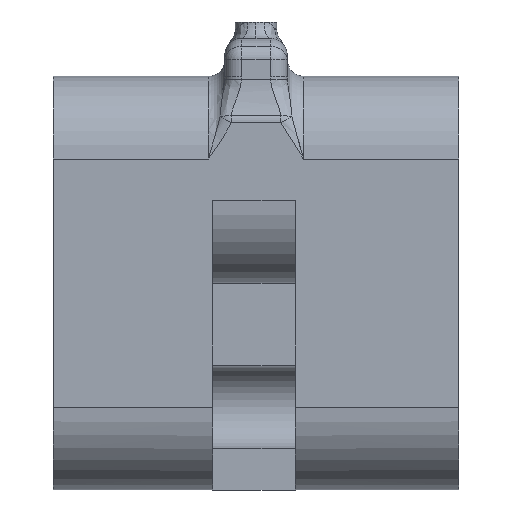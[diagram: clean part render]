
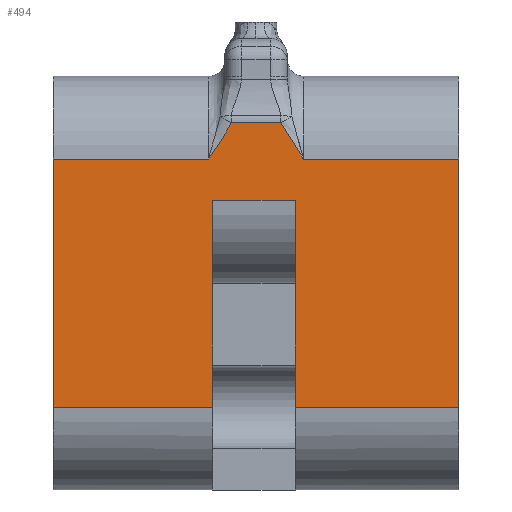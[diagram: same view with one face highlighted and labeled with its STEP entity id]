
A CAD part, front view. The second image highlights one B-rep face of the part: STEP entity #494.
In plain terms, the highlighted planar face has unit normal (0, -1, 0).
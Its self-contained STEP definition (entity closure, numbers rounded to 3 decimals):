
#110 = CARTESIAN_POINT ( 'NONE',  ( 28.243, -10., 32.181 ) ) ;
#115 = VERTEX_POINT ( 'NONE', #1654 ) ;
#188 = CARTESIAN_POINT ( 'NONE',  ( 49., -10., 29.345 ) ) ;
#259 = EDGE_CURVE ( 'NONE', #1880, #4710, #4178, .T. ) ;
#390 = CARTESIAN_POINT ( 'NONE',  ( 19.25, -10., -0.655 ) ) ;
#406 = DIRECTION ( 'NONE',  ( 0., 0., -1. ) ) ;
#482 = CARTESIAN_POINT ( 'NONE',  ( 30.25, -10., 29.345 ) ) ;
#494 = ADVANCED_FACE ( 'NONE', ( #1255 ), #2719, .F. ) ;
#531 = DIRECTION ( 'NONE',  ( -1., 0., 0. ) ) ;
#641 = CARTESIAN_POINT ( 'NONE',  ( 18.75, -10., 29.345 ) ) ;
#656 = CARTESIAN_POINT ( 'NONE',  ( 19.25, -10., 14.345 ) ) ;
#669 = VERTEX_POINT ( 'NONE', #2231 ) ;
#671 = ORIENTED_EDGE ( 'NONE', *, *, #1751, .T. ) ;
#687 = ORIENTED_EDGE ( 'NONE', *, *, #1184, .F. ) ;
#701 = ORIENTED_EDGE ( 'NONE', *, *, #1715, .F. ) ;
#867 = CARTESIAN_POINT ( 'NONE',  ( 29.25, -10., 14.345 ) ) ;
#896 = VECTOR ( 'NONE', #406, 1000. ) ;
#1102 = LINE ( 'NONE', #3932, #2811 ) ;
#1156 = LINE ( 'NONE', #2899, #1277 ) ;
#1184 = EDGE_CURVE ( 'NONE', #669, #2606, #2725, .T. ) ;
#1230 = CARTESIAN_POINT ( 'NONE',  ( 30.25, -10., 29.345 ) ) ;
#1255 = FACE_OUTER_BOUND ( 'NONE', #4703, .T. ) ;
#1276 = CARTESIAN_POINT ( 'NONE',  ( 49., -10., -0.655 ) ) ;
#1277 = VECTOR ( 'NONE', #3592, 1000. ) ;
#1285 = ORIENTED_EDGE ( 'NONE', *, *, #1675, .T. ) ;
#1381 = CARTESIAN_POINT ( 'NONE',  ( 21.527, -10., 33.727 ) ) ;
#1405 = CARTESIAN_POINT ( 'NONE',  ( 49., -10., 29.345 ) ) ;
#1433 = EDGE_CURVE ( 'NONE', #1954, #3858, #3478, .T. ) ;
#1469 = EDGE_CURVE ( 'NONE', #669, #3858, #2438, .T. ) ;
#1502 = VERTEX_POINT ( 'NONE', #2718 ) ;
#1506 = ORIENTED_EDGE ( 'NONE', *, *, #1469, .T. ) ;
#1568 = VECTOR ( 'NONE', #531, 1000. ) ;
#1599 = EDGE_CURVE ( 'NONE', #1880, #115, #1986, .T. ) ;
#1652 = ORIENTED_EDGE ( 'NONE', *, *, #259, .T. ) ;
#1654 = CARTESIAN_POINT ( 'NONE',  ( 49., -10., -0.655 ) ) ;
#1675 = EDGE_CURVE ( 'NONE', #4710, #4110, #2772, .T. ) ;
#1715 = EDGE_CURVE ( 'NONE', #115, #1954, #4276, .T. ) ;
#1732 = CARTESIAN_POINT ( 'NONE',  ( 21.527, -10., 33.727 ) ) ;
#1736 = VERTEX_POINT ( 'NONE', #3406 ) ;
#1751 = EDGE_CURVE ( 'NONE', #4110, #2814, #2527, .T. ) ;
#1840 = EDGE_CURVE ( 'NONE', #2814, #4041, #2340, .T. ) ;
#1880 = VERTEX_POINT ( 'NONE', #1405 ) ;
#1915 = EDGE_CURVE ( 'NONE', #1736, #1502, #1102, .T. ) ;
#1954 = VERTEX_POINT ( 'NONE', #2559 ) ;
#1981 = DIRECTION ( 'NONE',  ( -1., 0., 0. ) ) ;
#1986 = LINE ( 'NONE', #2986, #896 ) ;
#2076 = LINE ( 'NONE', #4075, #4694 ) ;
#2231 = CARTESIAN_POINT ( 'NONE',  ( 19.25, -10., 24.345 ) ) ;
#2297 = ORIENTED_EDGE ( 'NONE', *, *, #1915, .T. ) ;
#2323 = VECTOR ( 'NONE', #3401, 1000. ) ;
#2340 = B_SPLINE_CURVE_WITH_KNOTS ( 'NONE', 3,
 ( #1732, #3876, #2825, #641 ),
 .UNSPECIFIED., .F., .F.,
 ( 4, 4 ),
 ( 0.005, 0.01 ),
 .UNSPECIFIED. ) ;
#2344 = CARTESIAN_POINT ( 'NONE',  ( 49., -10., -0.655 ) ) ;
#2438 = LINE ( 'NONE', #4486, #2323 ) ;
#2483 = ORIENTED_EDGE ( 'NONE', *, *, #1433, .F. ) ;
#2527 = LINE ( 'NONE', #3063, #1568 ) ;
#2546 = VECTOR ( 'NONE', #3385, 1000. ) ;
#2559 = CARTESIAN_POINT ( 'NONE',  ( 29.25, -10., -0.655 ) ) ;
#2567 = CARTESIAN_POINT ( 'NONE',  ( 18.75, -10., 29.345 ) ) ;
#2606 = VERTEX_POINT ( 'NONE', #390 ) ;
#2678 = CARTESIAN_POINT ( 'NONE',  ( 29.248, -10., 30.763 ) ) ;
#2693 = CARTESIAN_POINT ( 'NONE',  ( 27.473, -10., 33.727 ) ) ;
#2718 = CARTESIAN_POINT ( 'NONE',  ( 0., -10., -0.655 ) ) ;
#2719 = PLANE ( 'NONE',  #3271 ) ;
#2725 = LINE ( 'NONE', #656, #4624 ) ;
#2772 = B_SPLINE_CURVE_WITH_KNOTS ( 'NONE', 3,
 ( #1230, #2678, #110, #2693 ),
 .UNSPECIFIED., .F., .F.,
 ( 4, 4 ),
 ( 0., 0.005 ),
 .UNSPECIFIED. ) ;
#2806 = DIRECTION ( 'NONE',  ( 0., 0., 1. ) ) ;
#2811 = VECTOR ( 'NONE', #3561, 1000. ) ;
#2814 = VERTEX_POINT ( 'NONE', #1381 ) ;
#2825 = CARTESIAN_POINT ( 'NONE',  ( 19.753, -10., 30.764 ) ) ;
#2899 = CARTESIAN_POINT ( 'NONE',  ( 49., -10., 29.345 ) ) ;
#2959 = CARTESIAN_POINT ( 'NONE',  ( 27.473, -10., 33.727 ) ) ;
#2986 = CARTESIAN_POINT ( 'NONE',  ( 49., -10., -0.655 ) ) ;
#3063 = CARTESIAN_POINT ( 'NONE',  ( 49., -10., 33.727 ) ) ;
#3106 = VECTOR ( 'NONE', #3388, 1000. ) ;
#3108 = ORIENTED_EDGE ( 'NONE', *, *, #1599, .F. ) ;
#3173 = DIRECTION ( 'NONE',  ( 0., 0., -1. ) ) ;
#3271 = AXIS2_PLACEMENT_3D ( 'NONE', #1276, #4244, #2806 ) ;
#3306 = VECTOR ( 'NONE', #1981, 1000. ) ;
#3385 = DIRECTION ( 'NONE',  ( 0., 0., 1. ) ) ;
#3388 = DIRECTION ( 'NONE',  ( -1., 0., 0. ) ) ;
#3401 = DIRECTION ( 'NONE',  ( 1., 0., 0. ) ) ;
#3406 = CARTESIAN_POINT ( 'NONE',  ( 0., -10., 29.345 ) ) ;
#3430 = CARTESIAN_POINT ( 'NONE',  ( 29.25, -10., 24.345 ) ) ;
#3478 = LINE ( 'NONE', #867, #2546 ) ;
#3505 = ORIENTED_EDGE ( 'NONE', *, *, #4373, .T. ) ;
#3561 = DIRECTION ( 'NONE',  ( 0., 0., -1. ) ) ;
#3592 = DIRECTION ( 'NONE',  ( -1., 0., 0. ) ) ;
#3858 = VERTEX_POINT ( 'NONE', #3430 ) ;
#3876 = CARTESIAN_POINT ( 'NONE',  ( 20.757, -10., 32.181 ) ) ;
#3932 = CARTESIAN_POINT ( 'NONE',  ( 0., -10., -0.655 ) ) ;
#4041 = VERTEX_POINT ( 'NONE', #2567 ) ;
#4075 = CARTESIAN_POINT ( 'NONE',  ( 49., -10., -0.655 ) ) ;
#4110 = VERTEX_POINT ( 'NONE', #2959 ) ;
#4156 = EDGE_CURVE ( 'NONE', #2606, #1502, #2076, .T. ) ;
#4162 = ORIENTED_EDGE ( 'NONE', *, *, #4156, .F. ) ;
#4178 = LINE ( 'NONE', #188, #3106 ) ;
#4244 = DIRECTION ( 'NONE',  ( 0., 1., 0. ) ) ;
#4276 = LINE ( 'NONE', #2344, #3306 ) ;
#4315 = ORIENTED_EDGE ( 'NONE', *, *, #1840, .T. ) ;
#4373 = EDGE_CURVE ( 'NONE', #4041, #1736, #1156, .T. ) ;
#4478 = DIRECTION ( 'NONE',  ( -1., 0., 0. ) ) ;
#4486 = CARTESIAN_POINT ( 'NONE',  ( 49., -10., 24.345 ) ) ;
#4624 = VECTOR ( 'NONE', #3173, 1000. ) ;
#4694 = VECTOR ( 'NONE', #4478, 1000. ) ;
#4703 = EDGE_LOOP ( 'NONE', ( #687, #1506, #2483, #701, #3108, #1652, #1285, #671, #4315, #3505, #2297, #4162 ) ) ;
#4710 = VERTEX_POINT ( 'NONE', #482 ) ;
